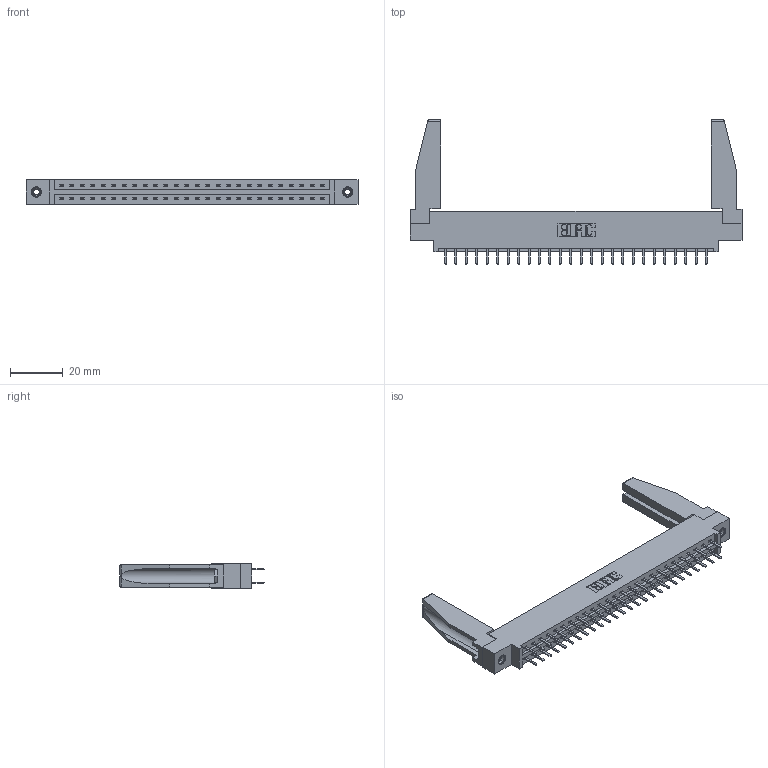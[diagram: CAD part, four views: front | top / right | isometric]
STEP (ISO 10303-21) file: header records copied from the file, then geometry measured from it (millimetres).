
FILE_DESCRIPTION (( 'STEP AP203' ), '1' );
FILE_NAME ('337-052-520-878.STEP', '2019-10-11T18:03:18', ( '' ), ( '' ), 'SwSTEP 2.0', 'SolidWorks 2016', '' );
FILE_SCHEMA (( 'CONFIG_CONTROL_DESIGN' ));
Length unit declared in the file: inch
Products named in the file (5): 337-052-520-878; 337 Part_0.170 Offset - 0.156 Dia-TI; 345-250-001_345-250-001-102; 345-292-001_345-293-120; 307-220-078
Assembly tree (57 placements, depth 2):
  337-052-520-878
    337 Part_0.170 Offset - 0.156 Dia-TI
    345-292-001_345-293-120  x52
    345-250-001_345-250-001-102  x2
    307-220-078  x2
Bounding box: 126.03 x 54.82 x 9.4 mm (x, y, z)
Volume: 16922.5 mm3; surface area: 18334.2 mm2
Topology: 57 solids, 57 shells, 3264 faces, 9441 edges, 6146 vertices
Faces by surface type: plane 2238, cylinder 1010, cone 12, torus 4
Entity records: 24914 total; most frequent: CARTESIAN_POINT 4224, ORIENTED_EDGE 4104, DIRECTION 3616, EDGE_CURVE 2052, VECTOR 1882, LINE 1882, VERTEX_POINT 1360, AXIS2_PLACEMENT_3D 867
